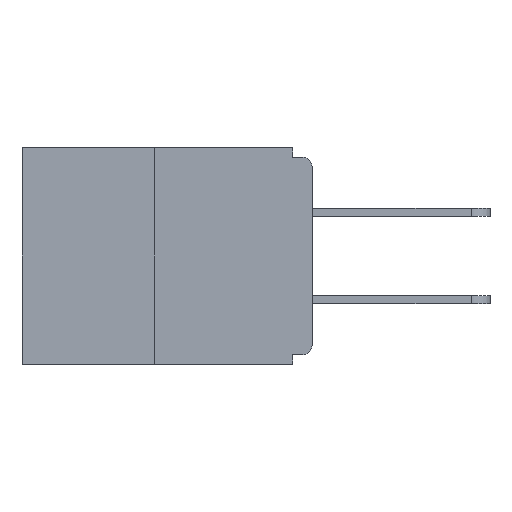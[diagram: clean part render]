
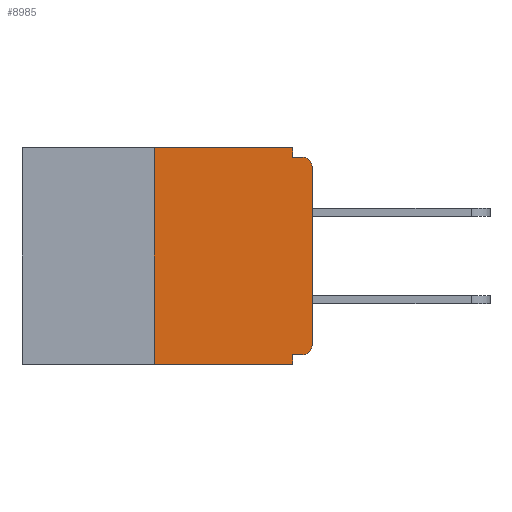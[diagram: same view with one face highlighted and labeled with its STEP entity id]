
A CAD part, left-side view. The second image highlights one B-rep face of the part: STEP entity #8985.
In plain terms, the highlighted planar face has unit normal (-1, 0, 0).
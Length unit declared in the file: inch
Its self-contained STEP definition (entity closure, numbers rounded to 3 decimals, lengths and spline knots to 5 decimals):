
#396 = CARTESIAN_POINT ( 'NONE',  ( 0., 0., -0.313 ) ) ;
#633 = EDGE_CURVE ( 'NONE', #7714, #27751, #9919, .T. ) ;
#809 = CARTESIAN_POINT ( 'NONE',  ( 0., 0.031, 0. ) ) ;
#1150 = VERTEX_POINT ( 'NONE', #13309 ) ;
#1163 = CARTESIAN_POINT ( 'NONE',  ( 0., 0.031, -0.015 ) ) ;
#1926 = VECTOR ( 'NONE', #29821, 39.37008 ) ;
#2091 = CIRCLE ( 'NONE', #18589, 0.015 ) ;
#2244 = VECTOR ( 'NONE', #8014, 39.37008 ) ;
#2254 = DIRECTION ( 'NONE',  ( 0., 0., -1. ) ) ;
#2403 = ORIENTED_EDGE ( 'NONE', *, *, #9141, .F. ) ;
#2613 = EDGE_CURVE ( 'NONE', #30842, #20964, #4037, .T. ) ;
#2838 = VECTOR ( 'NONE', #20879, 39.37008 ) ;
#3130 = ORIENTED_EDGE ( 'NONE', *, *, #27764, .F. ) ;
#3706 = CARTESIAN_POINT ( 'NONE',  ( 0., 0.031, -0.328 ) ) ;
#4037 = LINE ( 'NONE', #18303, #11264 ) ;
#4907 = VERTEX_POINT ( 'NONE', #1163 ) ;
#5203 = AXIS2_PLACEMENT_3D ( 'NONE', #25710, #11242, #30544 ) ;
#5373 = CARTESIAN_POINT ( 'NONE',  ( 0., 0.031, -0.343 ) ) ;
#5456 = ORIENTED_EDGE ( 'NONE', *, *, #2613, .F. ) ;
#5521 = LINE ( 'NONE', #8621, #16891 ) ;
#6276 = DIRECTION ( 'NONE',  ( 0., 0., -1. ) ) ;
#6490 = EDGE_CURVE ( 'NONE', #9095, #4907, #5521, .T. ) ;
#7051 = AXIS2_PLACEMENT_3D ( 'NONE', #24013, #9587, #2254 ) ;
#7565 = LINE ( 'NONE', #25016, #2244 ) ;
#7620 = EDGE_CURVE ( 'NONE', #27751, #15231, #2091, .T. ) ;
#7714 = VERTEX_POINT ( 'NONE', #396 ) ;
#8014 = DIRECTION ( 'NONE',  ( 0., -1., 0. ) ) ;
#8621 = CARTESIAN_POINT ( 'NONE',  ( 0., 0.031, 0. ) ) ;
#8985 = ADVANCED_FACE ( 'NONE', ( #19796 ), #16745, .F. ) ;
#9095 = VERTEX_POINT ( 'NONE', #809 ) ;
#9141 = EDGE_CURVE ( 'NONE', #19688, #1150, #30746, .T. ) ;
#9587 = DIRECTION ( 'NONE',  ( 1., 0., 0. ) ) ;
#9651 = EDGE_CURVE ( 'NONE', #30842, #7714, #16725, .T. ) ;
#9919 = LINE ( 'NONE', #27587, #1926 ) ;
#10148 = LINE ( 'NONE', #5373, #22966 ) ;
#10537 = ORIENTED_EDGE ( 'NONE', *, *, #15316, .T. ) ;
#11112 = DIRECTION ( 'NONE',  ( 0., 1., 0. ) ) ;
#11242 = DIRECTION ( 'NONE',  ( -1., 0., 0. ) ) ;
#11264 = VECTOR ( 'NONE', #11112, 39.37008 ) ;
#12673 = LINE ( 'NONE', #28229, #2838 ) ;
#12923 = CARTESIAN_POINT ( 'NONE',  ( 0., 0., -0.015 ) ) ;
#13221 = ORIENTED_EDGE ( 'NONE', *, *, #6490, .F. ) ;
#13309 = CARTESIAN_POINT ( 'NONE',  ( 0., 0.25, 0. ) ) ;
#13989 = DIRECTION ( 'NONE',  ( 0., 0., -1. ) ) ;
#14257 = ORIENTED_EDGE ( 'NONE', *, *, #26375, .F. ) ;
#15199 = ORIENTED_EDGE ( 'NONE', *, *, #7620, .T. ) ;
#15231 = VERTEX_POINT ( 'NONE', #17000 ) ;
#15316 = EDGE_CURVE ( 'NONE', #19688, #31159, #7565, .T. ) ;
#15516 = VECTOR ( 'NONE', #17923, 39.37008 ) ;
#15784 = CARTESIAN_POINT ( 'NONE',  ( 0., 0.25, -0.343 ) ) ;
#16725 = CIRCLE ( 'NONE', #5203, 0.015 ) ;
#16745 = PLANE ( 'NONE',  #7051 ) ;
#16891 = VECTOR ( 'NONE', #6276, 39.37008 ) ;
#17000 = CARTESIAN_POINT ( 'NONE',  ( 0., 0.015, -0.015 ) ) ;
#17250 = ORIENTED_EDGE ( 'NONE', *, *, #9651, .T. ) ;
#17923 = DIRECTION ( 'NONE',  ( 0., -1., 0. ) ) ;
#18031 = CARTESIAN_POINT ( 'NONE',  ( 0., 0.031, -0.343 ) ) ;
#18303 = CARTESIAN_POINT ( 'NONE',  ( 0., 0., -0.328 ) ) ;
#18462 = DIRECTION ( 'NONE',  ( 0., 0., 1. ) ) ;
#18589 = AXIS2_PLACEMENT_3D ( 'NONE', #24157, #20484, #13989 ) ;
#19688 = VERTEX_POINT ( 'NONE', #15784 ) ;
#19796 = FACE_OUTER_BOUND ( 'NONE', #24553, .T. ) ;
#20484 = DIRECTION ( 'NONE',  ( -1., 0., 0. ) ) ;
#20879 = DIRECTION ( 'NONE',  ( 0., -1., 0. ) ) ;
#20964 = VERTEX_POINT ( 'NONE', #3706 ) ;
#22966 = VECTOR ( 'NONE', #29608, 39.37008 ) ;
#23092 = CARTESIAN_POINT ( 'NONE',  ( 0., 0.25, 0. ) ) ;
#24013 = CARTESIAN_POINT ( 'NONE',  ( 0., 0.46, 0. ) ) ;
#24157 = CARTESIAN_POINT ( 'NONE',  ( 0., 0.015, -0.03 ) ) ;
#24553 = EDGE_LOOP ( 'NONE', ( #3130, #2403, #10537, #14257, #5456, #17250, #30176, #15199, #26799, #13221 ) ) ;
#24680 = VECTOR ( 'NONE', #18462, 39.37008 ) ;
#25016 = CARTESIAN_POINT ( 'NONE',  ( 0., 0.46, -0.343 ) ) ;
#25207 = EDGE_CURVE ( 'NONE', #4907, #15231, #26080, .T. ) ;
#25605 = CARTESIAN_POINT ( 'NONE',  ( 0., 0., -0.03 ) ) ;
#25710 = CARTESIAN_POINT ( 'NONE',  ( 0., 0.015, -0.313 ) ) ;
#26080 = LINE ( 'NONE', #12923, #15516 ) ;
#26375 = EDGE_CURVE ( 'NONE', #20964, #31159, #10148, .T. ) ;
#26799 = ORIENTED_EDGE ( 'NONE', *, *, #25207, .F. ) ;
#26900 = CARTESIAN_POINT ( 'NONE',  ( 0., 0.015, -0.328 ) ) ;
#27587 = CARTESIAN_POINT ( 'NONE',  ( 0., 0., 0. ) ) ;
#27751 = VERTEX_POINT ( 'NONE', #25605 ) ;
#27764 = EDGE_CURVE ( 'NONE', #1150, #9095, #12673, .T. ) ;
#28229 = CARTESIAN_POINT ( 'NONE',  ( 0., 0.46, 0. ) ) ;
#29608 = DIRECTION ( 'NONE',  ( 0., 0., -1. ) ) ;
#29821 = DIRECTION ( 'NONE',  ( 0., 0., 1. ) ) ;
#30176 = ORIENTED_EDGE ( 'NONE', *, *, #633, .T. ) ;
#30544 = DIRECTION ( 'NONE',  ( 0., 0., -1. ) ) ;
#30746 = LINE ( 'NONE', #23092, #24680 ) ;
#30842 = VERTEX_POINT ( 'NONE', #26900 ) ;
#31159 = VERTEX_POINT ( 'NONE', #18031 ) ;
